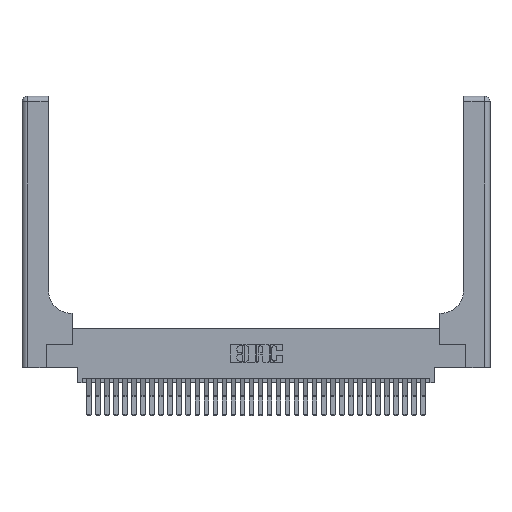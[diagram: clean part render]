
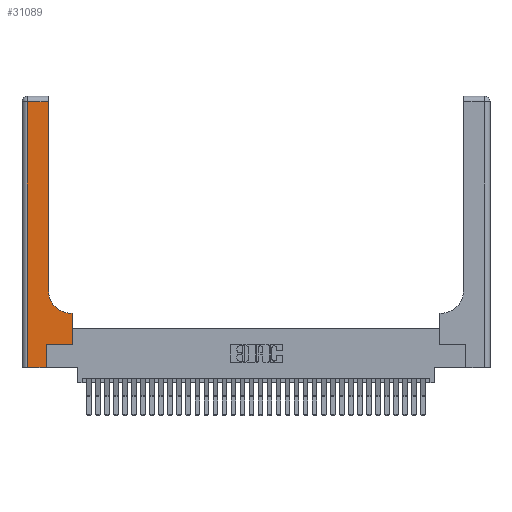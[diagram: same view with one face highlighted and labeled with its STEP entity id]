
A CAD part, top view. The second image highlights one B-rep face of the part: STEP entity #31089.
In plain terms, the highlighted planar face has unit normal (0, 0, 1).
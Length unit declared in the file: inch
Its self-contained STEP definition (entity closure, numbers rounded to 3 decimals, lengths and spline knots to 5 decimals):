
#996 = DIRECTION ( 'NONE',  ( -1., 0., 0. ) ) ;
#1242 = VERTEX_POINT ( 'NONE', #9893 ) ;
#1446 = DIRECTION ( 'NONE',  ( 1., 0., 0. ) ) ;
#2195 = ORIENTED_EDGE ( 'NONE', *, *, #16977, .T. ) ;
#3224 = AXIS2_PLACEMENT_3D ( 'NONE', #13638, #27713, #33153 ) ;
#3807 = CARTESIAN_POINT ( 'NONE',  ( 0.2915, 0.6, 0.37 ) ) ;
#4093 = VECTOR ( 'NONE', #1446, 39.37008 ) ;
#6496 = VERTEX_POINT ( 'NONE', #19067 ) ;
#6895 = CARTESIAN_POINT ( 'NONE',  ( 0.06, 2.94, 0.37 ) ) ;
#8676 = LINE ( 'NONE', #9571, #32493 ) ;
#9428 = CARTESIAN_POINT ( 'NONE',  ( 0.2915, 0.85, 0.37 ) ) ;
#9571 = CARTESIAN_POINT ( 'NONE',  ( 0.5585, 0.25, 0.37 ) ) ;
#9893 = CARTESIAN_POINT ( 'NONE',  ( 0.5585, 0.25, 0.37 ) ) ;
#10144 = VERTEX_POINT ( 'NONE', #9428 ) ;
#10180 = VERTEX_POINT ( 'NONE', #6895 ) ;
#10392 = CARTESIAN_POINT ( 'NONE',  ( 0.269, 0.25, 0.37 ) ) ;
#10842 = CIRCLE ( 'NONE', #3224, 0.25 ) ;
#11724 = VERTEX_POINT ( 'NONE', #15201 ) ;
#11937 = DIRECTION ( 'NONE',  ( -1., 0., 0. ) ) ;
#12420 = LINE ( 'NONE', #3807, #17198 ) ;
#13638 = CARTESIAN_POINT ( 'NONE',  ( 0.5415, 0.85, 0.37 ) ) ;
#13805 = EDGE_CURVE ( 'NONE', #34549, #19912, #32661, .T. ) ;
#14080 = AXIS2_PLACEMENT_3D ( 'NONE', #16653, #22309, #11937 ) ;
#15201 = CARTESIAN_POINT ( 'NONE',  ( 0.2915, 2.94, 0.37 ) ) ;
#16653 = CARTESIAN_POINT ( 'NONE',  ( 0., 3., 0.37 ) ) ;
#16977 = EDGE_CURVE ( 'NONE', #20487, #6496, #12420, .T. ) ;
#17198 = VECTOR ( 'NONE', #23187, 39.37008 ) ;
#17371 = VECTOR ( 'NONE', #996, 39.37008 ) ;
#17711 = ORIENTED_EDGE ( 'NONE', *, *, #24890, .T. ) ;
#17875 = CARTESIAN_POINT ( 'NONE',  ( 0.5585, 0.6, 0.37 ) ) ;
#18131 = LINE ( 'NONE', #20543, #29810 ) ;
#18617 = LINE ( 'NONE', #30077, #28038 ) ;
#19067 = CARTESIAN_POINT ( 'NONE',  ( 0.5415, 0.6, 0.37 ) ) ;
#19912 = VERTEX_POINT ( 'NONE', #31323 ) ;
#19921 = DIRECTION ( 'NONE',  ( 0., -1., 0. ) ) ;
#20148 = EDGE_CURVE ( 'NONE', #11724, #10180, #34671, .T. ) ;
#20487 = VERTEX_POINT ( 'NONE', #17875 ) ;
#20543 = CARTESIAN_POINT ( 'NONE',  ( 0.269, 0.25, 0.37 ) ) ;
#20593 = CARTESIAN_POINT ( 'NONE',  ( 0., 2.94, 0.37 ) ) ;
#20614 = DIRECTION ( 'NONE',  ( 0., 1., 0. ) ) ;
#20626 = ORIENTED_EDGE ( 'NONE', *, *, #13805, .T. ) ;
#22031 = EDGE_CURVE ( 'NONE', #10180, #34549, #18617, .T. ) ;
#22309 = DIRECTION ( 'NONE',  ( 0., 0., -1. ) ) ;
#23187 = DIRECTION ( 'NONE',  ( -1., 0., 0. ) ) ;
#24516 = CARTESIAN_POINT ( 'NONE',  ( 0.06, 0., 0.37 ) ) ;
#24587 = DIRECTION ( 'NONE',  ( 0., 1., 0. ) ) ;
#24890 = EDGE_CURVE ( 'NONE', #10144, #11724, #33095, .T. ) ;
#25747 = VECTOR ( 'NONE', #20614, 39.37008 ) ;
#26050 = EDGE_CURVE ( 'NONE', #19912, #35167, #30400, .T. ) ;
#26086 = DIRECTION ( 'NONE',  ( 1., 0., 0. ) ) ;
#26439 = PLANE ( 'NONE',  #14080 ) ;
#27713 = DIRECTION ( 'NONE',  ( 0., 0., -1. ) ) ;
#28038 = VECTOR ( 'NONE', #19921, 39.37008 ) ;
#28051 = EDGE_CURVE ( 'NONE', #1242, #20487, #8676, .T. ) ;
#28721 = ORIENTED_EDGE ( 'NONE', *, *, #31343, .T. ) ;
#28909 = CARTESIAN_POINT ( 'NONE',  ( 0.2915, 3., 0.37 ) ) ;
#29088 = CARTESIAN_POINT ( 'NONE',  ( 0., 0., 0.37 ) ) ;
#29310 = ORIENTED_EDGE ( 'NONE', *, *, #32356, .T. ) ;
#29810 = VECTOR ( 'NONE', #26086, 39.37008 ) ;
#29831 = ORIENTED_EDGE ( 'NONE', *, *, #26050, .T. ) ;
#29989 = VECTOR ( 'NONE', #24587, 39.37008 ) ;
#30077 = CARTESIAN_POINT ( 'NONE',  ( 0.06, 3., 0.37 ) ) ;
#30195 = CARTESIAN_POINT ( 'NONE',  ( 0.269, 0., 0.37 ) ) ;
#30400 = LINE ( 'NONE', #30195, #29989 ) ;
#31089 = ADVANCED_FACE ( 'NONE', ( #31606 ), #26439, .F. ) ;
#31323 = CARTESIAN_POINT ( 'NONE',  ( 0.269, 0., 0.37 ) ) ;
#31343 = EDGE_CURVE ( 'NONE', #6496, #10144, #10842, .T. ) ;
#31606 = FACE_OUTER_BOUND ( 'NONE', #35024, .T. ) ;
#32356 = EDGE_CURVE ( 'NONE', #35167, #1242, #18131, .T. ) ;
#32493 = VECTOR ( 'NONE', #34202, 39.37008 ) ;
#32542 = ORIENTED_EDGE ( 'NONE', *, *, #28051, .T. ) ;
#32661 = LINE ( 'NONE', #29088, #4093 ) ;
#33095 = LINE ( 'NONE', #28909, #25747 ) ;
#33153 = DIRECTION ( 'NONE',  ( 1., 0., 0. ) ) ;
#34202 = DIRECTION ( 'NONE',  ( 0., 1., 0. ) ) ;
#34549 = VERTEX_POINT ( 'NONE', #24516 ) ;
#34671 = LINE ( 'NONE', #20593, #17371 ) ;
#34944 = ORIENTED_EDGE ( 'NONE', *, *, #20148, .T. ) ;
#35024 = EDGE_LOOP ( 'NONE', ( #17711, #34944, #35576, #20626, #29831, #29310, #32542, #2195, #28721 ) ) ;
#35167 = VERTEX_POINT ( 'NONE', #10392 ) ;
#35576 = ORIENTED_EDGE ( 'NONE', *, *, #22031, .T. ) ;
